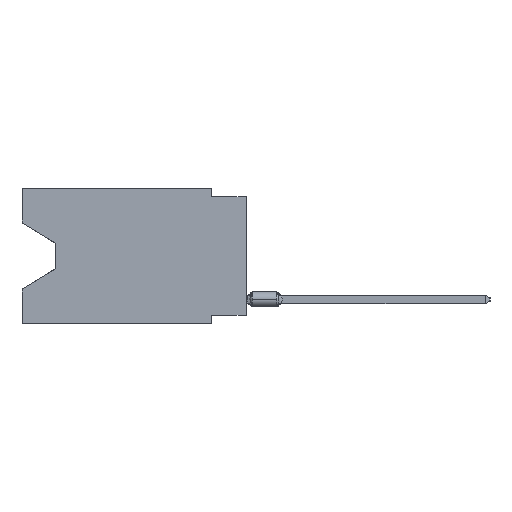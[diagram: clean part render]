
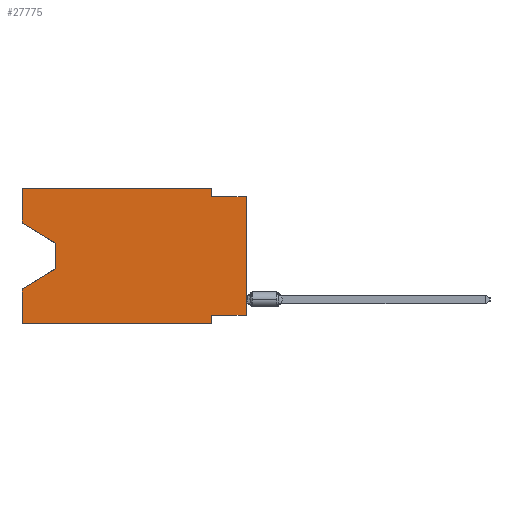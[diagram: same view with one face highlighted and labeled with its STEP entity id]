
A CAD part, left-side view. The second image highlights one B-rep face of the part: STEP entity #27775.
In plain terms, the highlighted planar face has unit normal (-1, 0, 0).
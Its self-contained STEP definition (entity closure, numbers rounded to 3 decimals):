
#46 = CARTESIAN_POINT ( 'NONE',  ( 0., 13.97, -5.893 ) ) ;
#526 = VERTEX_POINT ( 'NONE', #804 ) ;
#561 = VECTOR ( 'NONE', #22108, 1000. ) ;
#734 = VECTOR ( 'NONE', #11814, 1000. ) ;
#804 = CARTESIAN_POINT ( 'NONE',  ( 0., 2.54, -9.906 ) ) ;
#956 = EDGE_CURVE ( 'NONE', #28957, #25024, #24211, .T. ) ;
#1118 = AXIS2_PLACEMENT_3D ( 'NONE', #7713, #25734, #12226 ) ;
#1251 = DIRECTION ( 'NONE',  ( 0., -0.855, -0.519 ) ) ;
#1342 = VERTEX_POINT ( 'NONE', #8836 ) ;
#1376 = LINE ( 'NONE', #14339, #561 ) ;
#1513 = CARTESIAN_POINT ( 'NONE',  ( 0., 16.383, 0. ) ) ;
#2191 = EDGE_CURVE ( 'NONE', #2695, #29673, #7138, .T. ) ;
#2231 = CARTESIAN_POINT ( 'NONE',  ( 0., 2.54, -0.635 ) ) ;
#2324 = VECTOR ( 'NONE', #14515, 1000. ) ;
#2577 = DIRECTION ( 'NONE',  ( 0., 1., 0. ) ) ;
#2695 = VERTEX_POINT ( 'NONE', #7090 ) ;
#2976 = LINE ( 'NONE', #22724, #28745 ) ;
#3351 = EDGE_LOOP ( 'NONE', ( #19064, #3689, #13149, #14607, #32882, #29426, #25422, #7938, #30893, #27034, #24140, #25176 ) ) ;
#3689 = ORIENTED_EDGE ( 'NONE', *, *, #26855, .T. ) ;
#4394 = VECTOR ( 'NONE', #19219, 1000. ) ;
#4437 = VECTOR ( 'NONE', #27613, 1000. ) ;
#5288 = VECTOR ( 'NONE', #23001, 1000. ) ;
#5594 = VERTEX_POINT ( 'NONE', #15236 ) ;
#5966 = EDGE_CURVE ( 'NONE', #2695, #18592, #9970, .T. ) ;
#6203 = CARTESIAN_POINT ( 'NONE',  ( 0., 16.383, -7.36 ) ) ;
#6420 = DIRECTION ( 'NONE',  ( 0., 0., -1. ) ) ;
#6928 = EDGE_CURVE ( 'NONE', #24633, #18592, #2976, .T. ) ;
#7090 = CARTESIAN_POINT ( 'NONE',  ( 0., 0., -9.271 ) ) ;
#7138 = LINE ( 'NONE', #33097, #28478 ) ;
#7713 = CARTESIAN_POINT ( 'NONE',  ( 0., 16.383, 0. ) ) ;
#7938 = ORIENTED_EDGE ( 'NONE', *, *, #5966, .T. ) ;
#8836 = CARTESIAN_POINT ( 'NONE',  ( 0., 13.97, -4.013 ) ) ;
#9079 = CARTESIAN_POINT ( 'NONE',  ( 0., 16.383, -9.906 ) ) ;
#9970 = LINE ( 'NONE', #17547, #2324 ) ;
#10224 = FACE_OUTER_BOUND ( 'NONE', #3351, .T. ) ;
#11328 = EDGE_CURVE ( 'NONE', #29673, #526, #14129, .T. ) ;
#11814 = DIRECTION ( 'NONE',  ( 0., 0., 1. ) ) ;
#12226 = DIRECTION ( 'NONE',  ( 0., 0., -1. ) ) ;
#13149 = ORIENTED_EDGE ( 'NONE', *, *, #17633, .T. ) ;
#13623 = VECTOR ( 'NONE', #1251, 1000. ) ;
#14049 = LINE ( 'NONE', #24356, #13623 ) ;
#14129 = LINE ( 'NONE', #32517, #4437 ) ;
#14339 = CARTESIAN_POINT ( 'NONE',  ( 0., 13.97, -4.013 ) ) ;
#14515 = DIRECTION ( 'NONE',  ( 0., 0., 1. ) ) ;
#14607 = ORIENTED_EDGE ( 'NONE', *, *, #14756, .F. ) ;
#14660 = EDGE_CURVE ( 'NONE', #25024, #24633, #24296, .T. ) ;
#14756 = EDGE_CURVE ( 'NONE', #23435, #25275, #29497, .T. ) ;
#15236 = CARTESIAN_POINT ( 'NONE',  ( 0., 13.97, -5.893 ) ) ;
#15276 = PLANE ( 'NONE',  #1118 ) ;
#17321 = CARTESIAN_POINT ( 'NONE',  ( 0., 16.383, -9.906 ) ) ;
#17547 = CARTESIAN_POINT ( 'NONE',  ( 0., 0., 0. ) ) ;
#17633 = EDGE_CURVE ( 'NONE', #5594, #25275, #30905, .T. ) ;
#18169 = CARTESIAN_POINT ( 'NONE',  ( 0., 0., -0.635 ) ) ;
#18592 = VERTEX_POINT ( 'NONE', #18169 ) ;
#19064 = ORIENTED_EDGE ( 'NONE', *, *, #30801, .T. ) ;
#19219 = DIRECTION ( 'NONE',  ( 0., 0., 1. ) ) ;
#19552 = CARTESIAN_POINT ( 'NONE',  ( 0., 2.54, 0. ) ) ;
#22108 = DIRECTION ( 'NONE',  ( 0., 0., -1. ) ) ;
#22402 = LINE ( 'NONE', #17321, #29749 ) ;
#22724 = CARTESIAN_POINT ( 'NONE',  ( 0., 0., -0.635 ) ) ;
#23001 = DIRECTION ( 'NONE',  ( 0., 0.855, -0.519 ) ) ;
#23435 = VERTEX_POINT ( 'NONE', #9079 ) ;
#24140 = ORIENTED_EDGE ( 'NONE', *, *, #956, .F. ) ;
#24211 = LINE ( 'NONE', #27069, #31706 ) ;
#24296 = LINE ( 'NONE', #19552, #25385 ) ;
#24356 = CARTESIAN_POINT ( 'NONE',  ( 0., 16.383, -2.546 ) ) ;
#24633 = VERTEX_POINT ( 'NONE', #2231 ) ;
#25024 = VERTEX_POINT ( 'NONE', #32532 ) ;
#25176 = ORIENTED_EDGE ( 'NONE', *, *, #32576, .F. ) ;
#25275 = VERTEX_POINT ( 'NONE', #6203 ) ;
#25385 = VECTOR ( 'NONE', #6420, 1000. ) ;
#25422 = ORIENTED_EDGE ( 'NONE', *, *, #2191, .F. ) ;
#25734 = DIRECTION ( 'NONE',  ( 1., 0., 0. ) ) ;
#25739 = DIRECTION ( 'NONE',  ( 0., -1., 0. ) ) ;
#26106 = CARTESIAN_POINT ( 'NONE',  ( 0., 2.54, -9.271 ) ) ;
#26855 = EDGE_CURVE ( 'NONE', #1342, #5594, #1376, .T. ) ;
#27034 = ORIENTED_EDGE ( 'NONE', *, *, #14660, .F. ) ;
#27069 = CARTESIAN_POINT ( 'NONE',  ( 0., 16.383, 0. ) ) ;
#27613 = DIRECTION ( 'NONE',  ( 0., 0., -1. ) ) ;
#27775 = ADVANCED_FACE ( 'NONE', ( #10224 ), #15276, .F. ) ;
#28478 = VECTOR ( 'NONE', #2577, 1000. ) ;
#28745 = VECTOR ( 'NONE', #25739, 1000. ) ;
#28957 = VERTEX_POINT ( 'NONE', #29358 ) ;
#29358 = CARTESIAN_POINT ( 'NONE',  ( 0., 16.383, 0. ) ) ;
#29426 = ORIENTED_EDGE ( 'NONE', *, *, #11328, .F. ) ;
#29497 = LINE ( 'NONE', #1513, #4394 ) ;
#29673 = VERTEX_POINT ( 'NONE', #26106 ) ;
#29699 = CARTESIAN_POINT ( 'NONE',  ( 0., 16.383, 0. ) ) ;
#29749 = VECTOR ( 'NONE', #30813, 1000. ) ;
#29903 = DIRECTION ( 'NONE',  ( 0., -1., 0. ) ) ;
#30801 = EDGE_CURVE ( 'NONE', #32046, #1342, #14049, .T. ) ;
#30813 = DIRECTION ( 'NONE',  ( 0., -1., 0. ) ) ;
#30893 = ORIENTED_EDGE ( 'NONE', *, *, #6928, .F. ) ;
#30905 = LINE ( 'NONE', #46, #5288 ) ;
#31687 = EDGE_CURVE ( 'NONE', #23435, #526, #22402, .T. ) ;
#31706 = VECTOR ( 'NONE', #29903, 1000. ) ;
#32046 = VERTEX_POINT ( 'NONE', #32989 ) ;
#32517 = CARTESIAN_POINT ( 'NONE',  ( 0., 2.54, -9.906 ) ) ;
#32532 = CARTESIAN_POINT ( 'NONE',  ( 0., 2.54, 0. ) ) ;
#32566 = LINE ( 'NONE', #29699, #734 ) ;
#32576 = EDGE_CURVE ( 'NONE', #32046, #28957, #32566, .T. ) ;
#32882 = ORIENTED_EDGE ( 'NONE', *, *, #31687, .T. ) ;
#32989 = CARTESIAN_POINT ( 'NONE',  ( 0., 16.383, -2.546 ) ) ;
#33097 = CARTESIAN_POINT ( 'NONE',  ( 0., 0., -9.271 ) ) ;
